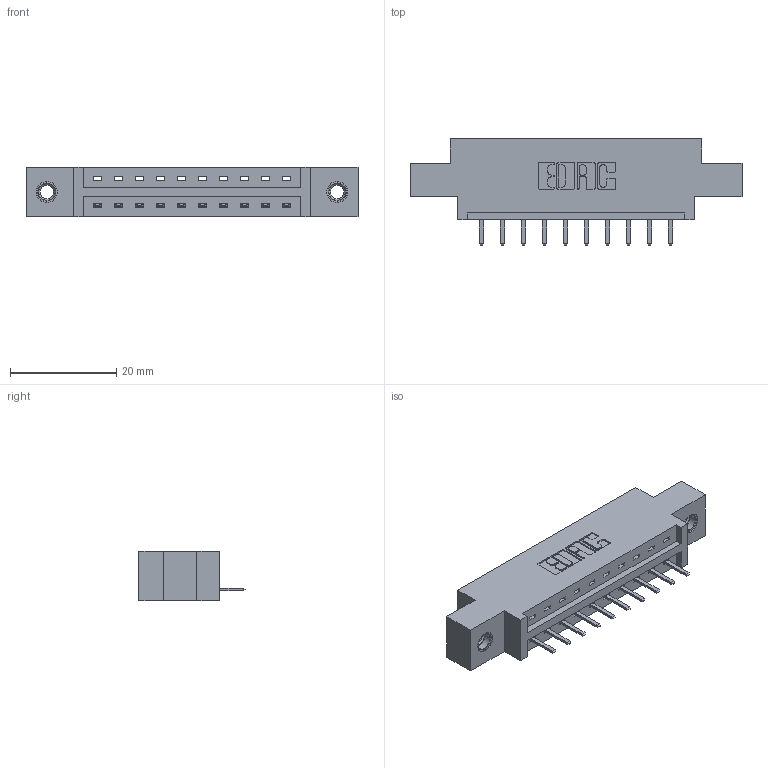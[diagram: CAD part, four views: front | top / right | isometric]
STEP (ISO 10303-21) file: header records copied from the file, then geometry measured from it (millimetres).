
FILE_DESCRIPTION (( 'STEP AP203' ), '1' );
FILE_NAME ('387-010-520-607.STEP', '2019-10-02T11:01:59', ( '' ), ( '' ), 'SwSTEP 2.0', 'SolidWorks 2016', '' );
FILE_SCHEMA (( 'CONFIG_CONTROL_DESIGN' ));
Length unit declared in the file: inch
Products named in the file (4): 345-292-001_345-293-120; 345-250-001_345-250-005-103; 337 Part_0.170 Offset - 0.156 Dia-TI; 387-010-520-607
Assembly tree (13 placements, depth 2):
  387-010-520-607
    337 Part_0.170 Offset - 0.156 Dia-TI
    345-292-001_345-293-120  x10
    345-250-001_345-250-005-103  x2
Bounding box: 62.64 x 20.02 x 9.4 mm (x, y, z)
Volume: 5949.8 mm3; surface area: 6004.5 mm2
Topology: 13 solids, 13 shells, 838 faces, 2419 edges, 1578 vertices
Faces by surface type: plane 586, cylinder 236, cone 12, torus 4
Entity records: 13004 total; most frequent: CARTESIAN_POINT 2255, ORIENTED_EDGE 2182, DIRECTION 1985, EDGE_CURVE 1091, VECTOR 939, LINE 939, VERTEX_POINT 720, AXIS2_PLACEMENT_3D 523
